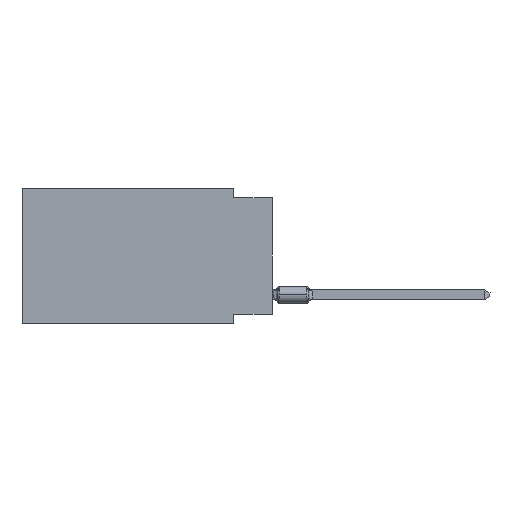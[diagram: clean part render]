
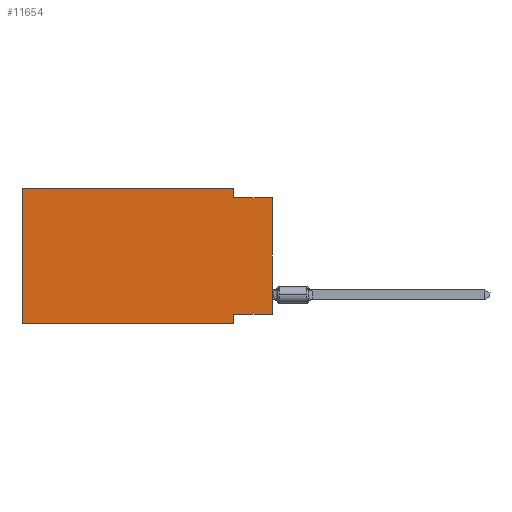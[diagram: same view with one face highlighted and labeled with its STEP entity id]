
A CAD part, left-side view. The second image highlights one B-rep face of the part: STEP entity #11654.
In plain terms, the highlighted planar face has unit normal (-1, 0, 0).
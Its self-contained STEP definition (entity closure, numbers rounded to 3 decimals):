
#25 = VERTEX_POINT ( 'NONE', #3685 ) ;
#1056 = VERTEX_POINT ( 'NONE', #8564 ) ;
#1073 = VERTEX_POINT ( 'NONE', #10805 ) ;
#1835 = VECTOR ( 'NONE', #29977, 1000. ) ;
#3108 = VERTEX_POINT ( 'NONE', #19146 ) ;
#3685 = CARTESIAN_POINT ( 'NONE',  ( 0., 16.383, 0. ) ) ;
#3996 = LINE ( 'NONE', #18500, #14705 ) ;
#4001 = LINE ( 'NONE', #18814, #25034 ) ;
#4008 = CARTESIAN_POINT ( 'NONE',  ( 0., 0., -0.635 ) ) ;
#4043 = EDGE_CURVE ( 'NONE', #6039, #1073, #4001, .T. ) ;
#5287 = DIRECTION ( 'NONE',  ( 1., 0., 0. ) ) ;
#6039 = VERTEX_POINT ( 'NONE', #17280 ) ;
#6588 = EDGE_CURVE ( 'NONE', #27866, #15359, #10541, .T. ) ;
#8301 = DIRECTION ( 'NONE',  ( 0., -1., 0. ) ) ;
#8434 = LINE ( 'NONE', #20869, #18233 ) ;
#8564 = CARTESIAN_POINT ( 'NONE',  ( 0., 16.383, -8.89 ) ) ;
#8791 = LINE ( 'NONE', #4008, #12985 ) ;
#8898 = DIRECTION ( 'NONE',  ( 0., 1., 0. ) ) ;
#9025 = CARTESIAN_POINT ( 'NONE',  ( 0., 2.54, -8.255 ) ) ;
#9077 = VECTOR ( 'NONE', #14561, 1000. ) ;
#9212 = CARTESIAN_POINT ( 'NONE',  ( 0., 0., -8.255 ) ) ;
#9849 = LINE ( 'NONE', #19577, #17029 ) ;
#9944 = EDGE_CURVE ( 'NONE', #1056, #15359, #9849, .T. ) ;
#10530 = ORIENTED_EDGE ( 'NONE', *, *, #9944, .T. ) ;
#10541 = LINE ( 'NONE', #25371, #1835 ) ;
#10805 = CARTESIAN_POINT ( 'NONE',  ( 0., 2.54, -0.635 ) ) ;
#10944 = VERTEX_POINT ( 'NONE', #24786 ) ;
#11654 = ADVANCED_FACE ( 'NONE', ( #29508 ), #18748, .F. ) ;
#11706 = CARTESIAN_POINT ( 'NONE',  ( 0., 16.383, 0. ) ) ;
#12331 = EDGE_CURVE ( 'NONE', #10944, #3108, #8434, .T. ) ;
#12985 = VECTOR ( 'NONE', #8301, 1000. ) ;
#13282 = EDGE_CURVE ( 'NONE', #10944, #27866, #31044, .T. ) ;
#13537 = ORIENTED_EDGE ( 'NONE', *, *, #22973, .F. ) ;
#13564 = DIRECTION ( 'NONE',  ( 0., -1., 0. ) ) ;
#14150 = CARTESIAN_POINT ( 'NONE',  ( 0., 2.54, -8.89 ) ) ;
#14413 = EDGE_CURVE ( 'NONE', #1073, #3108, #8791, .T. ) ;
#14546 = DIRECTION ( 'NONE',  ( 0., 0., -1. ) ) ;
#14561 = DIRECTION ( 'NONE',  ( 0., 0., 1. ) ) ;
#14705 = VECTOR ( 'NONE', #13564, 1000. ) ;
#15359 = VERTEX_POINT ( 'NONE', #14150 ) ;
#16814 = AXIS2_PLACEMENT_3D ( 'NONE', #16937, #5287, #14546 ) ;
#16937 = CARTESIAN_POINT ( 'NONE',  ( 0., 16.383, 0. ) ) ;
#17029 = VECTOR ( 'NONE', #29293, 1000. ) ;
#17280 = CARTESIAN_POINT ( 'NONE',  ( 0., 2.54, 0. ) ) ;
#18233 = VECTOR ( 'NONE', #27876, 1000. ) ;
#18500 = CARTESIAN_POINT ( 'NONE',  ( 0., 16.383, 0. ) ) ;
#18748 = PLANE ( 'NONE',  #16814 ) ;
#18814 = CARTESIAN_POINT ( 'NONE',  ( 0., 2.54, 0. ) ) ;
#19143 = ORIENTED_EDGE ( 'NONE', *, *, #30312, .F. ) ;
#19146 = CARTESIAN_POINT ( 'NONE',  ( 0., 0., -0.635 ) ) ;
#19577 = CARTESIAN_POINT ( 'NONE',  ( 0., 16.383, -8.89 ) ) ;
#20610 = ORIENTED_EDGE ( 'NONE', *, *, #14413, .F. ) ;
#20869 = CARTESIAN_POINT ( 'NONE',  ( 0., 0., 0. ) ) ;
#22964 = EDGE_LOOP ( 'NONE', ( #25550, #20610, #27242, #19143, #13537, #10530, #23443, #31441 ) ) ;
#22973 = EDGE_CURVE ( 'NONE', #1056, #25, #26056, .T. ) ;
#23443 = ORIENTED_EDGE ( 'NONE', *, *, #6588, .F. ) ;
#23775 = DIRECTION ( 'NONE',  ( 0., 0., -1. ) ) ;
#24786 = CARTESIAN_POINT ( 'NONE',  ( 0., 0., -8.255 ) ) ;
#25034 = VECTOR ( 'NONE', #23775, 1000. ) ;
#25371 = CARTESIAN_POINT ( 'NONE',  ( 0., 2.54, -8.89 ) ) ;
#25550 = ORIENTED_EDGE ( 'NONE', *, *, #12331, .T. ) ;
#26056 = LINE ( 'NONE', #11706, #9077 ) ;
#27242 = ORIENTED_EDGE ( 'NONE', *, *, #4043, .F. ) ;
#27866 = VERTEX_POINT ( 'NONE', #9025 ) ;
#27876 = DIRECTION ( 'NONE',  ( 0., 0., 1. ) ) ;
#28702 = VECTOR ( 'NONE', #8898, 1000. ) ;
#29293 = DIRECTION ( 'NONE',  ( 0., -1., 0. ) ) ;
#29508 = FACE_OUTER_BOUND ( 'NONE', #22964, .T. ) ;
#29977 = DIRECTION ( 'NONE',  ( 0., 0., -1. ) ) ;
#30312 = EDGE_CURVE ( 'NONE', #25, #6039, #3996, .T. ) ;
#31044 = LINE ( 'NONE', #9212, #28702 ) ;
#31441 = ORIENTED_EDGE ( 'NONE', *, *, #13282, .F. ) ;
